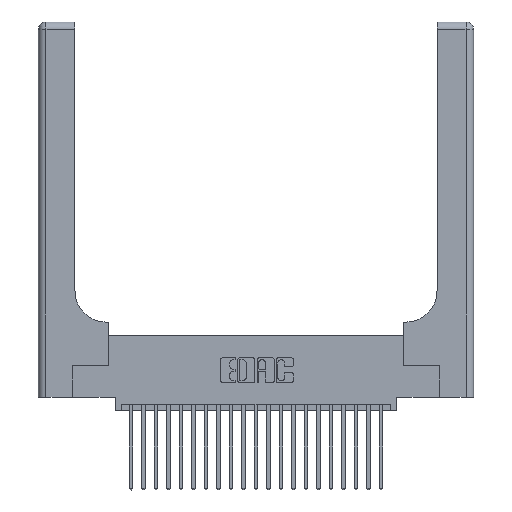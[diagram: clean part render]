
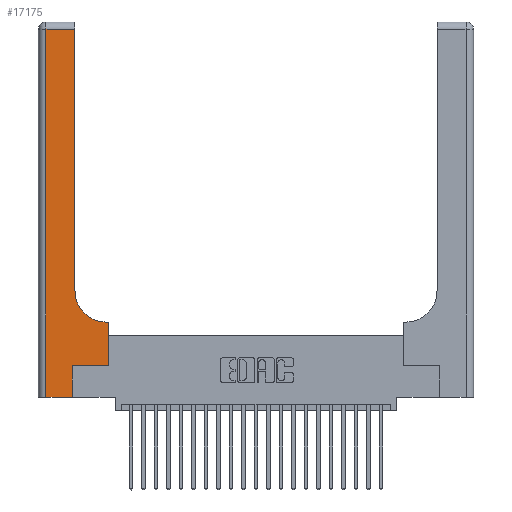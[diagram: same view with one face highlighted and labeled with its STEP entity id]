
A CAD part, top view. The second image highlights one B-rep face of the part: STEP entity #17175.
In plain terms, the highlighted planar face has unit normal (0, 0, 1).
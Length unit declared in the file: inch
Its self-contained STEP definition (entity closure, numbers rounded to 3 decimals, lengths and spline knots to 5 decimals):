
#218 = EDGE_LOOP ( 'NONE', ( #18525, #10112, #23822, #22676, #9078, #14687, #3704, #5918, #12232 ) ) ;
#654 = VERTEX_POINT ( 'NONE', #6228 ) ;
#762 = LINE ( 'NONE', #15818, #17749 ) ;
#769 = EDGE_CURVE ( 'NONE', #2582, #5788, #2673, .T. ) ;
#884 = VERTEX_POINT ( 'NONE', #4057 ) ;
#1325 = CARTESIAN_POINT ( 'NONE',  ( 0.2915, 0.85, 0.37 ) ) ;
#1339 = CARTESIAN_POINT ( 'NONE',  ( 0.06, 0., 0.37 ) ) ;
#1777 = AXIS2_PLACEMENT_3D ( 'NONE', #11018, #9069, #18700 ) ;
#2136 = EDGE_CURVE ( 'NONE', #22441, #13857, #14433, .T. ) ;
#2265 = EDGE_CURVE ( 'NONE', #22135, #654, #23428, .T. ) ;
#2328 = VERTEX_POINT ( 'NONE', #12433 ) ;
#2582 = VERTEX_POINT ( 'NONE', #1339 ) ;
#2673 = LINE ( 'NONE', #4303, #20837 ) ;
#3704 = ORIENTED_EDGE ( 'NONE', *, *, #2265, .T. ) ;
#3739 = DIRECTION ( 'NONE',  ( -1., 0., 0. ) ) ;
#3843 = VECTOR ( 'NONE', #14759, 39.37008 ) ;
#4057 = CARTESIAN_POINT ( 'NONE',  ( 0.269, 0.25, 0.37 ) ) ;
#4303 = CARTESIAN_POINT ( 'NONE',  ( 0., 0., 0.37 ) ) ;
#4375 = LINE ( 'NONE', #4551, #14200 ) ;
#4400 = VECTOR ( 'NONE', #7483, 39.37008 ) ;
#4427 = LINE ( 'NONE', #8209, #3843 ) ;
#4551 = CARTESIAN_POINT ( 'NONE',  ( 0.2915, 3., 0.37 ) ) ;
#4606 = AXIS2_PLACEMENT_3D ( 'NONE', #13097, #22831, #3739 ) ;
#5214 = CARTESIAN_POINT ( 'NONE',  ( 0.06, 3., 0.37 ) ) ;
#5788 = VERTEX_POINT ( 'NONE', #23649 ) ;
#5918 = ORIENTED_EDGE ( 'NONE', *, *, #18104, .T. ) ;
#6228 = CARTESIAN_POINT ( 'NONE',  ( 0.5585, 0.6, 0.37 ) ) ;
#6458 = CARTESIAN_POINT ( 'NONE',  ( 0.269, 0.25, 0.37 ) ) ;
#6709 = DIRECTION ( 'NONE',  ( 1., 0., 0. ) ) ;
#7268 = VECTOR ( 'NONE', #6709, 39.37008 ) ;
#7321 = CARTESIAN_POINT ( 'NONE',  ( 0.269, 0., 0.37 ) ) ;
#7483 = DIRECTION ( 'NONE',  ( 0., 1., 0. ) ) ;
#8209 = CARTESIAN_POINT ( 'NONE',  ( 0.2915, 0.6, 0.37 ) ) ;
#8485 = LINE ( 'NONE', #7321, #4400 ) ;
#9069 = DIRECTION ( 'NONE',  ( 0., 0., -1. ) ) ;
#9078 = ORIENTED_EDGE ( 'NONE', *, *, #18179, .T. ) ;
#9675 = EDGE_CURVE ( 'NONE', #10647, #2328, #762, .T. ) ;
#10112 = ORIENTED_EDGE ( 'NONE', *, *, #9675, .T. ) ;
#10280 = DIRECTION ( 'NONE',  ( 0., 1., 0. ) ) ;
#10647 = VERTEX_POINT ( 'NONE', #20471 ) ;
#10833 = CARTESIAN_POINT ( 'NONE',  ( 0.5585, 0.25, 0.37 ) ) ;
#11018 = CARTESIAN_POINT ( 'NONE',  ( 0.5415, 0.85, 0.37 ) ) ;
#11801 = CARTESIAN_POINT ( 'NONE',  ( 0.5415, 0.6, 0.37 ) ) ;
#12029 = DIRECTION ( 'NONE',  ( 1., 0., 0. ) ) ;
#12232 = ORIENTED_EDGE ( 'NONE', *, *, #2136, .T. ) ;
#12409 = LINE ( 'NONE', #5214, #20490 ) ;
#12433 = CARTESIAN_POINT ( 'NONE',  ( 0.06, 2.94, 0.37 ) ) ;
#12925 = PLANE ( 'NONE',  #4606 ) ;
#13097 = CARTESIAN_POINT ( 'NONE',  ( 0., 3., 0.37 ) ) ;
#13857 = VERTEX_POINT ( 'NONE', #1325 ) ;
#13877 = DIRECTION ( 'NONE',  ( -1., 0., 0. ) ) ;
#14046 = CARTESIAN_POINT ( 'NONE',  ( 0.5585, 0.25, 0.37 ) ) ;
#14200 = VECTOR ( 'NONE', #10280, 39.37008 ) ;
#14433 = CIRCLE ( 'NONE', #1777, 0.25 ) ;
#14687 = ORIENTED_EDGE ( 'NONE', *, *, #23159, .T. ) ;
#14759 = DIRECTION ( 'NONE',  ( -1., 0., 0. ) ) ;
#15012 = LINE ( 'NONE', #6458, #7268 ) ;
#15122 = EDGE_CURVE ( 'NONE', #2328, #2582, #12409, .T. ) ;
#15818 = CARTESIAN_POINT ( 'NONE',  ( 0., 2.94, 0.37 ) ) ;
#16394 = FACE_OUTER_BOUND ( 'NONE', #218, .T. ) ;
#16540 = VECTOR ( 'NONE', #21578, 39.37008 ) ;
#16808 = DIRECTION ( 'NONE',  ( 0., -1., 0. ) ) ;
#17175 = ADVANCED_FACE ( 'NONE', ( #16394 ), #12925, .F. ) ;
#17749 = VECTOR ( 'NONE', #13877, 39.37008 ) ;
#18104 = EDGE_CURVE ( 'NONE', #654, #22441, #4427, .T. ) ;
#18179 = EDGE_CURVE ( 'NONE', #5788, #884, #8485, .T. ) ;
#18525 = ORIENTED_EDGE ( 'NONE', *, *, #18567, .T. ) ;
#18567 = EDGE_CURVE ( 'NONE', #13857, #10647, #4375, .T. ) ;
#18700 = DIRECTION ( 'NONE',  ( 1., 0., 0. ) ) ;
#20471 = CARTESIAN_POINT ( 'NONE',  ( 0.2915, 2.94, 0.37 ) ) ;
#20490 = VECTOR ( 'NONE', #16808, 39.37008 ) ;
#20837 = VECTOR ( 'NONE', #12029, 39.37008 ) ;
#21578 = DIRECTION ( 'NONE',  ( 0., 1., 0. ) ) ;
#22135 = VERTEX_POINT ( 'NONE', #10833 ) ;
#22441 = VERTEX_POINT ( 'NONE', #11801 ) ;
#22676 = ORIENTED_EDGE ( 'NONE', *, *, #769, .T. ) ;
#22831 = DIRECTION ( 'NONE',  ( 0., 0., -1. ) ) ;
#23159 = EDGE_CURVE ( 'NONE', #884, #22135, #15012, .T. ) ;
#23428 = LINE ( 'NONE', #14046, #16540 ) ;
#23649 = CARTESIAN_POINT ( 'NONE',  ( 0.269, 0., 0.37 ) ) ;
#23822 = ORIENTED_EDGE ( 'NONE', *, *, #15122, .T. ) ;
